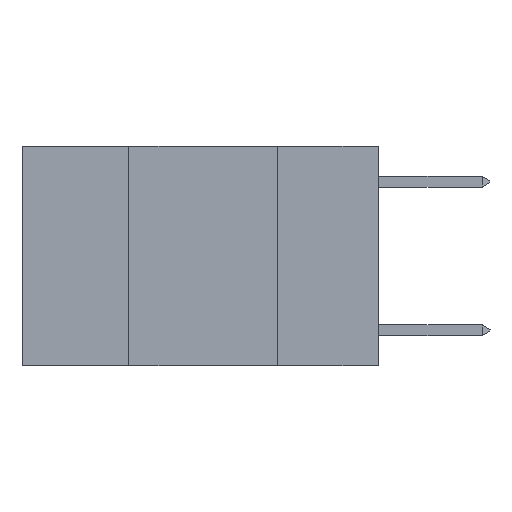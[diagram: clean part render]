
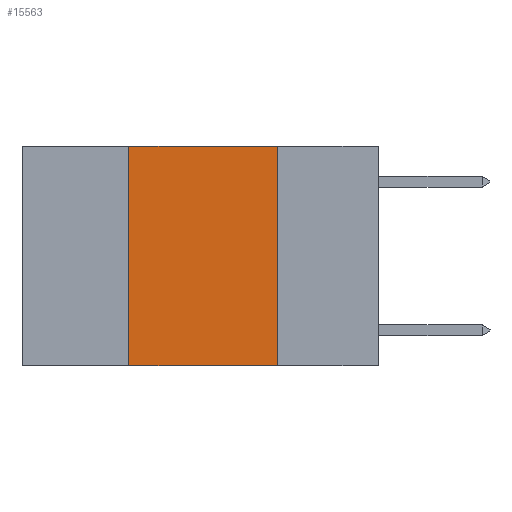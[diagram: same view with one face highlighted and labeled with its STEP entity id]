
A CAD part, left-side view. The second image highlights one B-rep face of the part: STEP entity #15563.
In plain terms, the highlighted planar face has unit normal (-1, 0, 0).
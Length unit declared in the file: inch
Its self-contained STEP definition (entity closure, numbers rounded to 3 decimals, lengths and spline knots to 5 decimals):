
#845 = CARTESIAN_POINT ( 'NONE',  ( 0., 0.42, 0. ) ) ;
#1826 = CARTESIAN_POINT ( 'NONE',  ( 0., 0.6, 0. ) ) ;
#2195 = CARTESIAN_POINT ( 'NONE',  ( 0., 0.42, 0. ) ) ;
#2227 = EDGE_LOOP ( 'NONE', ( #5554, #5761, #6595, #6966 ) ) ;
#2424 = DIRECTION ( 'NONE',  ( 0., -1., 0. ) ) ;
#3648 = VERTEX_POINT ( 'NONE', #4952 ) ;
#4295 = DIRECTION ( 'NONE',  ( 1., 0., 0. ) ) ;
#4952 = CARTESIAN_POINT ( 'NONE',  ( 0., 0.42, -0.37 ) ) ;
#5554 = ORIENTED_EDGE ( 'NONE', *, *, #23390, .F. ) ;
#5761 = ORIENTED_EDGE ( 'NONE', *, *, #29062, .F. ) ;
#5782 = EDGE_CURVE ( 'NONE', #3648, #9778, #12913, .T. ) ;
#6595 = ORIENTED_EDGE ( 'NONE', *, *, #5782, .F. ) ;
#6966 = ORIENTED_EDGE ( 'NONE', *, *, #11082, .T. ) ;
#7138 = CARTESIAN_POINT ( 'NONE',  ( 0., 0.6, 0. ) ) ;
#9778 = VERTEX_POINT ( 'NONE', #845 ) ;
#9861 = CARTESIAN_POINT ( 'NONE',  ( 0., 0.17, 0. ) ) ;
#11082 = EDGE_CURVE ( 'NONE', #3648, #23984, #22428, .T. ) ;
#12703 = VECTOR ( 'NONE', #27482, 39.37008 ) ;
#12913 = LINE ( 'NONE', #2195, #12703 ) ;
#13403 = VECTOR ( 'NONE', #19064, 39.37008 ) ;
#14119 = LINE ( 'NONE', #9861, #13403 ) ;
#14504 = CARTESIAN_POINT ( 'NONE',  ( 0., 0.17, -0.37 ) ) ;
#15157 = LINE ( 'NONE', #7138, #26462 ) ;
#15563 = ADVANCED_FACE ( 'NONE', ( #25544 ), #15897, .F. ) ;
#15897 = PLANE ( 'NONE',  #27392 ) ;
#16354 = VECTOR ( 'NONE', #26717, 39.37008 ) ;
#17711 = CARTESIAN_POINT ( 'NONE',  ( 0., 0.6, -0.37 ) ) ;
#19064 = DIRECTION ( 'NONE',  ( 0., 0., -1. ) ) ;
#20555 = DIRECTION ( 'NONE',  ( 0., 0., -1. ) ) ;
#22428 = LINE ( 'NONE', #17711, #16354 ) ;
#22881 = CARTESIAN_POINT ( 'NONE',  ( 0., 0.17, 0. ) ) ;
#23390 = EDGE_CURVE ( 'NONE', #24402, #23984, #14119, .T. ) ;
#23984 = VERTEX_POINT ( 'NONE', #14504 ) ;
#24402 = VERTEX_POINT ( 'NONE', #22881 ) ;
#25544 = FACE_OUTER_BOUND ( 'NONE', #2227, .T. ) ;
#26462 = VECTOR ( 'NONE', #2424, 39.37008 ) ;
#26717 = DIRECTION ( 'NONE',  ( 0., -1., 0. ) ) ;
#27392 = AXIS2_PLACEMENT_3D ( 'NONE', #1826, #4295, #20555 ) ;
#27482 = DIRECTION ( 'NONE',  ( 0., 0., 1. ) ) ;
#29062 = EDGE_CURVE ( 'NONE', #9778, #24402, #15157, .T. ) ;
